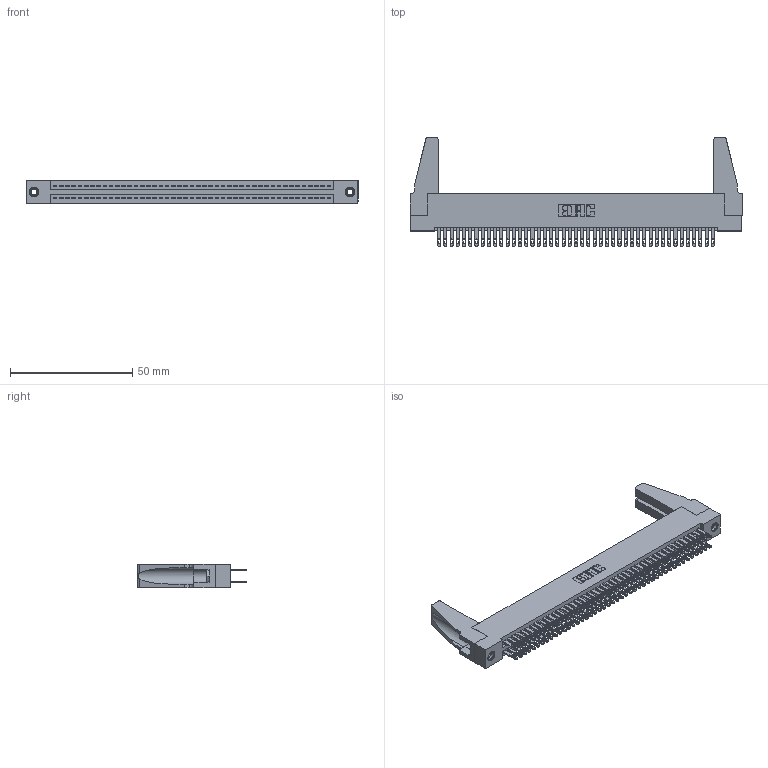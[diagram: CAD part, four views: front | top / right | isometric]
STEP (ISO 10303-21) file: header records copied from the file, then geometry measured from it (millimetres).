
FILE_DESCRIPTION (( 'STEP AP203' ), '1' );
FILE_NAME ('345-090-500-288.STEP', '2019-11-01T14:29:06', ( '' ), ( '' ), 'SwSTEP 2.0', 'SolidWorks 2016', '' );
FILE_SCHEMA (( 'CONFIG_CONTROL_DESIGN' ));
Length unit declared in the file: inch
Products named in the file (5): 345-090-500-288; 345 Part_Flush Mounting Lugs - 0.156 Dia-TH; 345-220-078_345-220-088; 345-292-001_345-293-100; 345-250-001_345-250-001-102
Assembly tree (95 placements, depth 2):
  345-090-500-288
    345 Part_Flush Mounting Lugs - 0.156 Dia-TH
    345-292-001_345-293-100  x90
    345-250-001_345-250-001-102  x2
    345-220-078_345-220-088  x2
Bounding box: 135.53 x 44.37 x 9.4 mm (x, y, z)
Volume: 16721.3 mm3; surface area: 24007.4 mm2
Topology: 95 solids, 95 shells, 4390 faces, 13345 edges, 8886 vertices
Faces by surface type: plane 2582, cylinder 1792, cone 12, torus 4
Entity records: 36982 total; most frequent: CARTESIAN_POINT 6190, ORIENTED_EDGE 6084, DIRECTION 5462, EDGE_CURVE 3042, LINE 2684, VECTOR 2684, VERTEX_POINT 2022, AXIS2_PLACEMENT_3D 1389
